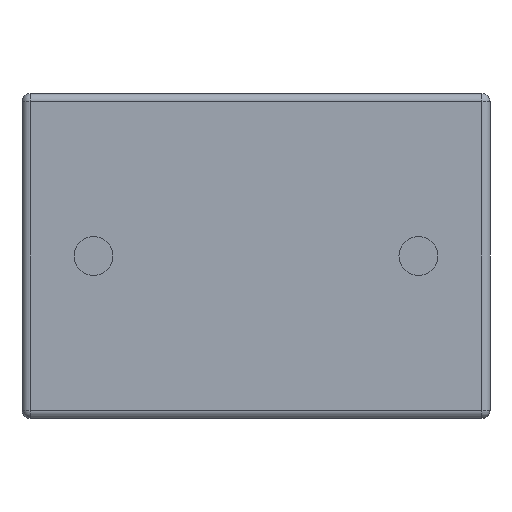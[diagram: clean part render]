
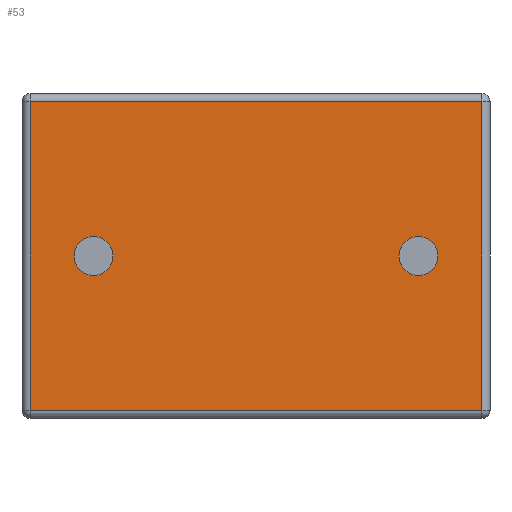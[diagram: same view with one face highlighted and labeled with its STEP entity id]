
A CAD part, front view. The second image highlights one B-rep face of the part: STEP entity #53.
In plain terms, the highlighted planar face has unit normal (0, -1, 0).
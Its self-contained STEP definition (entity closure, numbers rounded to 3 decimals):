
#53=ADVANCED_FACE('',(#323,#325,#327),#329,.T.);
#323=FACE_BOUND('',#324,.T.);
#324=EDGE_LOOP('',(#541,#542,#543,#544));
#325=FACE_BOUND('',#326,.T.);
#326=EDGE_LOOP('',(#545));
#327=FACE_BOUND('',#328,.T.);
#328=EDGE_LOOP('',(#546));
#329=PLANE('',#330);
#330=AXIS2_PLACEMENT_3D('',#331,#332,#333);
#331=CARTESIAN_POINT('',(-3.6,0.,-2.5));
#332=DIRECTION('',(0.,-1.,0.));
#333=DIRECTION('',(1.,0.,0.));
#541=ORIENTED_EDGE('',*,*,#645,.T.);
#542=ORIENTED_EDGE('',*,*,#646,.T.);
#543=ORIENTED_EDGE('',*,*,#647,.F.);
#544=ORIENTED_EDGE('',*,*,#648,.F.);
#545=ORIENTED_EDGE('',*,*,#649,.F.);
#546=ORIENTED_EDGE('',*,*,#650,.F.);
#645=EDGE_CURVE('',#697,#698,#699,.T.);
#646=EDGE_CURVE('',#698,#700,#701,.T.);
#647=EDGE_CURVE('',#702,#700,#703,.T.);
#648=EDGE_CURVE('',#697,#702,#704,.T.);
#649=EDGE_CURVE('',#705,#705,#706,.T.);
#650=EDGE_CURVE('',#707,#707,#708,.T.);
#697=VERTEX_POINT('',#777);
#698=VERTEX_POINT('',#778);
#699=LINE('',#779,#780);
#700=VERTEX_POINT('',#782);
#701=LINE('',#783,#784);
#702=VERTEX_POINT('',#786);
#703=LINE('',#787,#788);
#704=LINE('',#790,#791);
#705=VERTEX_POINT('',#793);
#706=CIRCLE('',#794,0.3);
#707=VERTEX_POINT('',#798);
#708=CIRCLE('',#799,0.3);
#777=CARTESIAN_POINT('',(-3.475,0.,-2.375));
#778=CARTESIAN_POINT('',(3.475,0.,-2.375));
#779=CARTESIAN_POINT('',(-3.475,0.,-2.375));
#780=VECTOR('',#781,1.);
#781=DIRECTION('',(1.,0.,0.));
#782=CARTESIAN_POINT('',(3.475,0.,2.375));
#783=CARTESIAN_POINT('',(3.475,0.,-2.375));
#784=VECTOR('',#785,1.);
#785=DIRECTION('',(0.,0.,1.));
#786=CARTESIAN_POINT('',(-3.475,0.,2.375));
#787=CARTESIAN_POINT('',(-3.475,0.,2.375));
#788=VECTOR('',#789,1.);
#789=DIRECTION('',(1.,0.,0.));
#790=CARTESIAN_POINT('',(-3.475,0.,-2.375));
#791=VECTOR('',#792,1.);
#792=DIRECTION('',(0.,0.,1.));
#793=CARTESIAN_POINT('',(-2.2,0.,0.));
#794=AXIS2_PLACEMENT_3D('',#795,#796,#797);
#795=CARTESIAN_POINT('',(-2.5,0.,0.));
#796=DIRECTION('',(0.,-1.,0.));
#797=DIRECTION('',(1.,0.,0.));
#798=CARTESIAN_POINT('',(2.8,0.,0.));
#799=AXIS2_PLACEMENT_3D('',#800,#801,#802);
#800=CARTESIAN_POINT('',(2.5,0.,0.));
#801=DIRECTION('',(0.,-1.,0.));
#802=DIRECTION('',(1.,0.,0.));
